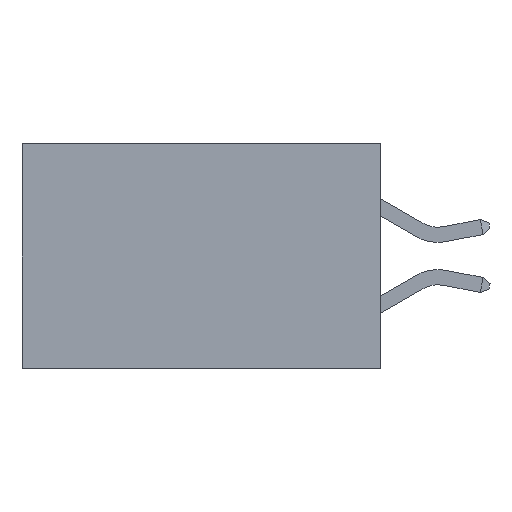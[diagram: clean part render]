
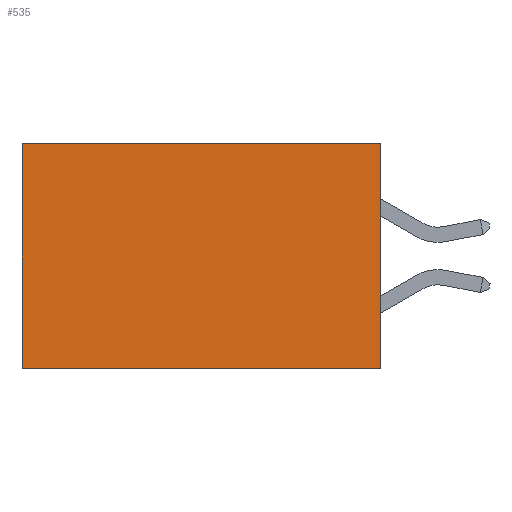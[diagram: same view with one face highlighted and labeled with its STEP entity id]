
A CAD part, left-side view. The second image highlights one B-rep face of the part: STEP entity #535.
In plain terms, the highlighted planar face has unit normal (-1, 0, 0).
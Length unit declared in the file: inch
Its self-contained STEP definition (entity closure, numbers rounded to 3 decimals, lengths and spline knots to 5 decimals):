
#2 = CARTESIAN_POINT ( 'NONE',  ( 0.277, 0., 0. ) ) ;
#27 = DIRECTION ( 'NONE',  ( 0., 1., 0. ) ) ;
#28 = ORIENTED_EDGE ( 'NONE', *, *, #875, .F. ) ;
#535 = ADVANCED_FACE ( 'NONE', ( #16815 ), #21571, .F. ) ;
#610 = EDGE_CURVE ( 'NONE', #11431, #15555, #15697, .T. ) ;
#875 = EDGE_CURVE ( 'NONE', #15555, #15816, #1008, .T. ) ;
#1008 = LINE ( 'NONE', #14836, #19548 ) ;
#1454 = DIRECTION ( 'NONE',  ( 0., 0., -1. ) ) ;
#2067 = CARTESIAN_POINT ( 'NONE',  ( 0.277, 0., -0.37 ) ) ;
#4579 = VECTOR ( 'NONE', #27, 39.37008 ) ;
#4586 = EDGE_CURVE ( 'NONE', #11431, #11071, #9360, .T. ) ;
#9148 = VECTOR ( 'NONE', #18888, 39.37008 ) ;
#9349 = EDGE_LOOP ( 'NONE', ( #14478, #28, #17275, #14761 ) ) ;
#9360 = LINE ( 'NONE', #2, #4579 ) ;
#9656 = CARTESIAN_POINT ( 'NONE',  ( 0.277, 0., -0.37 ) ) ;
#9984 = CARTESIAN_POINT ( 'NONE',  ( 0.277, 0.59, -0.37 ) ) ;
#11071 = VERTEX_POINT ( 'NONE', #16056 ) ;
#11157 = CARTESIAN_POINT ( 'NONE',  ( 0.277, 0., -0.37 ) ) ;
#11431 = VERTEX_POINT ( 'NONE', #13449 ) ;
#13449 = CARTESIAN_POINT ( 'NONE',  ( 0.277, 0., 0. ) ) ;
#13888 = CARTESIAN_POINT ( 'NONE',  ( 0.277, 0.59, -0.37 ) ) ;
#14286 = DIRECTION ( 'NONE',  ( 0., 0., -1. ) ) ;
#14478 = ORIENTED_EDGE ( 'NONE', *, *, #20852, .T. ) ;
#14497 = LINE ( 'NONE', #9984, #9148 ) ;
#14761 = ORIENTED_EDGE ( 'NONE', *, *, #4586, .T. ) ;
#14836 = CARTESIAN_POINT ( 'NONE',  ( 0.277, 0., -0.37 ) ) ;
#15555 = VERTEX_POINT ( 'NONE', #9656 ) ;
#15697 = LINE ( 'NONE', #11157, #16248 ) ;
#15816 = VERTEX_POINT ( 'NONE', #13888 ) ;
#16056 = CARTESIAN_POINT ( 'NONE',  ( 0.277, 0.59, 0. ) ) ;
#16128 = AXIS2_PLACEMENT_3D ( 'NONE', #2067, #21316, #14286 ) ;
#16248 = VECTOR ( 'NONE', #1454, 39.37008 ) ;
#16815 = FACE_OUTER_BOUND ( 'NONE', #9349, .T. ) ;
#17275 = ORIENTED_EDGE ( 'NONE', *, *, #610, .F. ) ;
#18813 = DIRECTION ( 'NONE',  ( 0., 1., 0. ) ) ;
#18888 = DIRECTION ( 'NONE',  ( 0., 0., -1. ) ) ;
#19548 = VECTOR ( 'NONE', #18813, 39.37008 ) ;
#20852 = EDGE_CURVE ( 'NONE', #11071, #15816, #14497, .T. ) ;
#21316 = DIRECTION ( 'NONE',  ( 1., 0., 0. ) ) ;
#21571 = PLANE ( 'NONE',  #16128 ) ;
